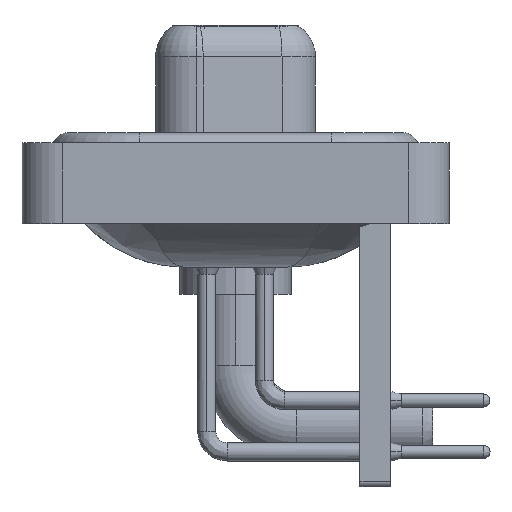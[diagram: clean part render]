
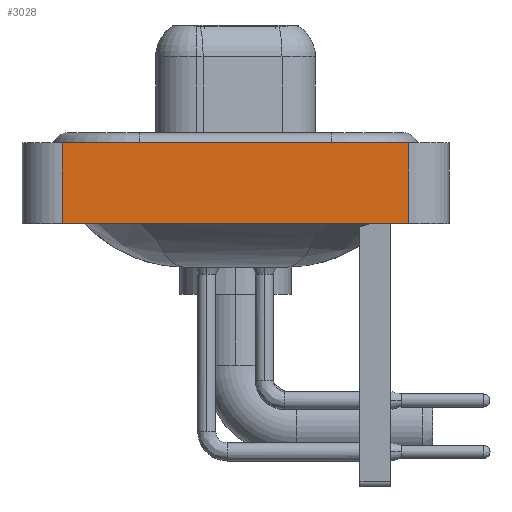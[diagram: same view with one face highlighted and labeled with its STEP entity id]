
A CAD part, left-side view. The second image highlights one B-rep face of the part: STEP entity #3028.
In plain terms, the highlighted planar face has unit normal (-1, 0, 0).
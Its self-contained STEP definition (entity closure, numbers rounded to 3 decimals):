
#340 = VERTEX_POINT ( 'NONE', #17102 ) ;
#389 = DIRECTION ( 'NONE',  ( 0., 0., 1. ) ) ;
#902 = CARTESIAN_POINT ( 'NONE',  ( -7.25, -8.55, -3.6 ) ) ;
#933 = DIRECTION ( 'NONE',  ( 0., -1., 0. ) ) ;
#1155 = LINE ( 'NONE', #15527, #16703 ) ;
#2107 = DIRECTION ( 'NONE',  ( 0., -1., 0. ) ) ;
#2386 = DIRECTION ( 'NONE',  ( 0., 0., 1. ) ) ;
#2816 = CARTESIAN_POINT ( 'NONE',  ( -7.25, 8.55, 0.4 ) ) ;
#2910 = EDGE_CURVE ( 'NONE', #12319, #14841, #1155, .T. ) ;
#3028 = ADVANCED_FACE ( 'NONE', ( #11542 ), #6503, .T. ) ;
#3252 = DIRECTION ( 'NONE',  ( -1., 0., 0. ) ) ;
#3522 = CARTESIAN_POINT ( 'NONE',  ( -7.25, -8.55, 0.4 ) ) ;
#4225 = EDGE_CURVE ( 'NONE', #12319, #340, #17830, .T. ) ;
#4309 = CARTESIAN_POINT ( 'NONE',  ( -7.25, -8.55, 0.4 ) ) ;
#5626 = VECTOR ( 'NONE', #933, 1000. ) ;
#5701 = ORIENTED_EDGE ( 'NONE', *, *, #2910, .F. ) ;
#6340 = AXIS2_PLACEMENT_3D ( 'NONE', #14661, #3252, #389 ) ;
#6503 = PLANE ( 'NONE',  #6340 ) ;
#7405 = ORIENTED_EDGE ( 'NONE', *, *, #4225, .T. ) ;
#8050 = VECTOR ( 'NONE', #2386, 1000. ) ;
#8108 = CARTESIAN_POINT ( 'NONE',  ( -7.25, 8.55, -3.6 ) ) ;
#9423 = VECTOR ( 'NONE', #2107, 1000. ) ;
#9571 = DIRECTION ( 'NONE',  ( 0., 0., 1. ) ) ;
#10474 = EDGE_CURVE ( 'NONE', #340, #19326, #16744, .T. ) ;
#11542 = FACE_OUTER_BOUND ( 'NONE', #14054, .T. ) ;
#11821 = EDGE_CURVE ( 'NONE', #14841, #19326, #15302, .T. ) ;
#11894 = CARTESIAN_POINT ( 'NONE',  ( -7.25, -8.55, -3.6 ) ) ;
#12319 = VERTEX_POINT ( 'NONE', #8108 ) ;
#13148 = ORIENTED_EDGE ( 'NONE', *, *, #10474, .T. ) ;
#14054 = EDGE_LOOP ( 'NONE', ( #13148, #14741, #5701, #7405 ) ) ;
#14661 = CARTESIAN_POINT ( 'NONE',  ( -7.25, -8.55, -3.6 ) ) ;
#14741 = ORIENTED_EDGE ( 'NONE', *, *, #11821, .F. ) ;
#14841 = VERTEX_POINT ( 'NONE', #2816 ) ;
#15302 = LINE ( 'NONE', #4309, #5626 ) ;
#15527 = CARTESIAN_POINT ( 'NONE',  ( -7.25, 8.55, -3.6 ) ) ;
#16703 = VECTOR ( 'NONE', #9571, 1000. ) ;
#16744 = LINE ( 'NONE', #902, #8050 ) ;
#17102 = CARTESIAN_POINT ( 'NONE',  ( -7.25, -8.55, -3.6 ) ) ;
#17830 = LINE ( 'NONE', #11894, #9423 ) ;
#19326 = VERTEX_POINT ( 'NONE', #3522 ) ;
